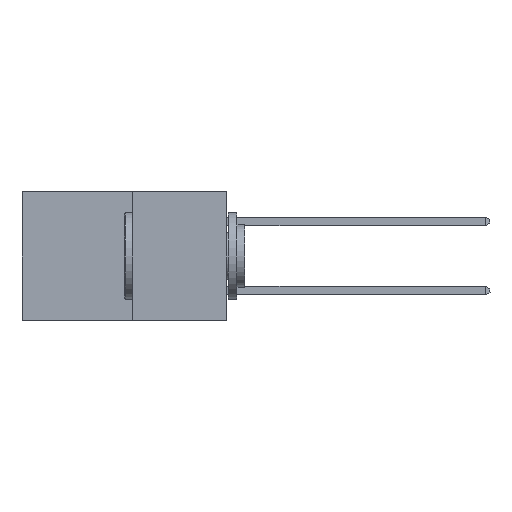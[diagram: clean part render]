
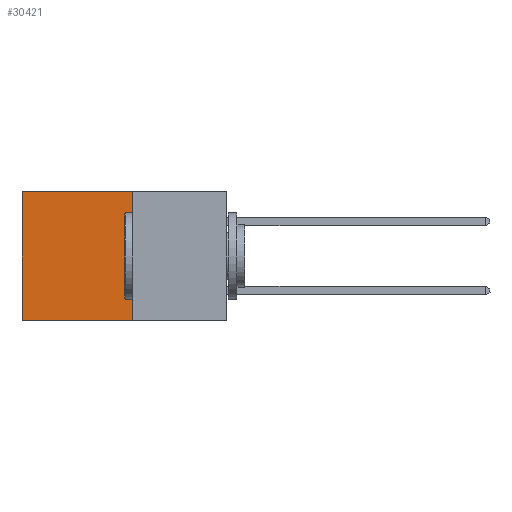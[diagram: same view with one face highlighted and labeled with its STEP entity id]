
A CAD part, left-side view. The second image highlights one B-rep face of the part: STEP entity #30421.
In plain terms, the highlighted planar face has unit normal (-1, 0, 0).
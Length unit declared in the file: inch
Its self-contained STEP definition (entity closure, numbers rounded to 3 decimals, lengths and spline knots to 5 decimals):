
#1525 = EDGE_CURVE ( 'NONE', #5534, #7759, #24321, .T. ) ;
#1798 = FACE_OUTER_BOUND ( 'NONE', #4906, .T. ) ;
#2169 = VERTEX_POINT ( 'NONE', #12083 ) ;
#2303 = CARTESIAN_POINT ( 'NONE',  ( 0.277, 0.27, -0.37 ) ) ;
#3342 = LINE ( 'NONE', #24361, #4143 ) ;
#4143 = VECTOR ( 'NONE', #9055, 39.37008 ) ;
#4906 = EDGE_LOOP ( 'NONE', ( #10993, #12707, #17401, #31118 ) ) ;
#5172 = CARTESIAN_POINT ( 'NONE',  ( 0.277, 0.27, -0.37 ) ) ;
#5534 = VERTEX_POINT ( 'NONE', #2303 ) ;
#6327 = VECTOR ( 'NONE', #12689, 39.37008 ) ;
#7717 = DIRECTION ( 'NONE',  ( 0., 0., -1. ) ) ;
#7759 = VERTEX_POINT ( 'NONE', #31171 ) ;
#8759 = LINE ( 'NONE', #24491, #14708 ) ;
#9055 = DIRECTION ( 'NONE',  ( 0., 1., 0. ) ) ;
#9441 = EDGE_CURVE ( 'NONE', #2169, #16904, #3342, .T. ) ;
#10993 = ORIENTED_EDGE ( 'NONE', *, *, #28116, .T. ) ;
#11764 = DIRECTION ( 'NONE',  ( 0., 0., -1. ) ) ;
#12083 = CARTESIAN_POINT ( 'NONE',  ( 0.277, 0.27, 0. ) ) ;
#12689 = DIRECTION ( 'NONE',  ( 0., 1., 0. ) ) ;
#12707 = ORIENTED_EDGE ( 'NONE', *, *, #1525, .F. ) ;
#14180 = CARTESIAN_POINT ( 'NONE',  ( 0.277, 0.59, 0. ) ) ;
#14708 = VECTOR ( 'NONE', #11764, 39.37008 ) ;
#15107 = CARTESIAN_POINT ( 'NONE',  ( 0.277, 0.27, -0.37 ) ) ;
#16904 = VERTEX_POINT ( 'NONE', #14180 ) ;
#17401 = ORIENTED_EDGE ( 'NONE', *, *, #23301, .F. ) ;
#18064 = VECTOR ( 'NONE', #30994, 39.37008 ) ;
#20415 = PLANE ( 'NONE',  #32097 ) ;
#23022 = DIRECTION ( 'NONE',  ( 1., 0., 0. ) ) ;
#23301 = EDGE_CURVE ( 'NONE', #2169, #5534, #24897, .T. ) ;
#23343 = CARTESIAN_POINT ( 'NONE',  ( 0.277, 0.27, -0.37 ) ) ;
#24321 = LINE ( 'NONE', #15107, #6327 ) ;
#24361 = CARTESIAN_POINT ( 'NONE',  ( 0.277, 0.27, 0. ) ) ;
#24491 = CARTESIAN_POINT ( 'NONE',  ( 0.277, 0.59, -0.37 ) ) ;
#24897 = LINE ( 'NONE', #23343, #18064 ) ;
#28116 = EDGE_CURVE ( 'NONE', #16904, #7759, #8759, .T. ) ;
#30421 = ADVANCED_FACE ( 'NONE', ( #1798 ), #20415, .F. ) ;
#30994 = DIRECTION ( 'NONE',  ( 0., 0., -1. ) ) ;
#31118 = ORIENTED_EDGE ( 'NONE', *, *, #9441, .T. ) ;
#31171 = CARTESIAN_POINT ( 'NONE',  ( 0.277, 0.59, -0.37 ) ) ;
#32097 = AXIS2_PLACEMENT_3D ( 'NONE', #5172, #23022, #7717 ) ;
